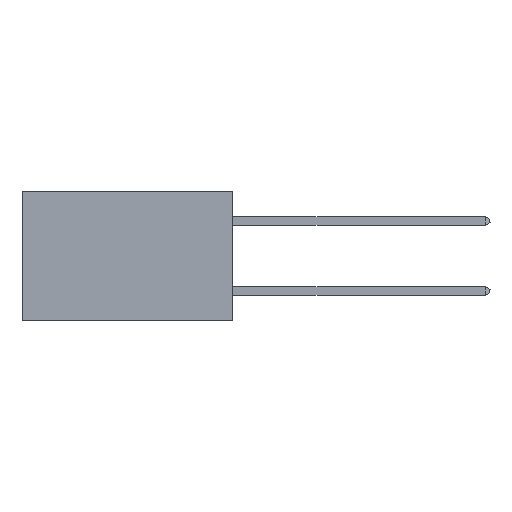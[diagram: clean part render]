
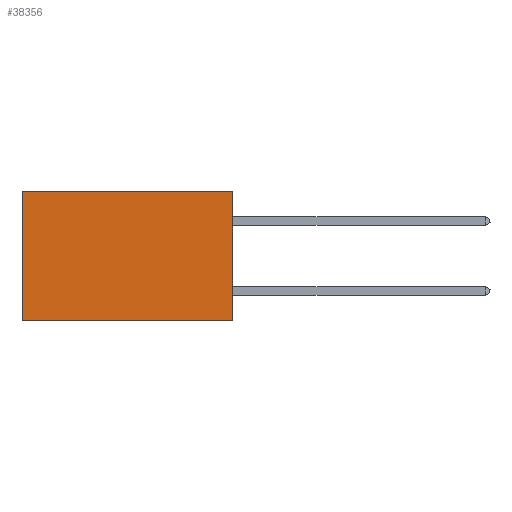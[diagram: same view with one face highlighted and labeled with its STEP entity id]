
A CAD part, left-side view. The second image highlights one B-rep face of the part: STEP entity #38356.
In plain terms, the highlighted planar face has unit normal (-1, 0, 0).
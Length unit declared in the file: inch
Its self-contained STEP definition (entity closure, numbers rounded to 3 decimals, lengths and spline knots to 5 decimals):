
#1992 = CARTESIAN_POINT ( 'NONE',  ( 0.2875, 0., -0.37 ) ) ;
#2346 = ORIENTED_EDGE ( 'NONE', *, *, #32950, .F. ) ;
#3374 = DIRECTION ( 'NONE',  ( 0., 1., 0. ) ) ;
#3600 = VECTOR ( 'NONE', #3374, 39.37008 ) ;
#3686 = VECTOR ( 'NONE', #34816, 39.37008 ) ;
#4096 = EDGE_CURVE ( 'NONE', #15948, #19096, #16349, .T. ) ;
#5787 = PLANE ( 'NONE',  #17945 ) ;
#6437 = CARTESIAN_POINT ( 'NONE',  ( 0.2875, 0., 0. ) ) ;
#8338 = VECTOR ( 'NONE', #11772, 39.37008 ) ;
#8766 = DIRECTION ( 'NONE',  ( 0., 0., -1. ) ) ;
#8863 = ORIENTED_EDGE ( 'NONE', *, *, #33765, .T. ) ;
#10231 = EDGE_CURVE ( 'NONE', #15948, #36506, #26880, .T. ) ;
#11419 = ORIENTED_EDGE ( 'NONE', *, *, #4096, .F. ) ;
#11712 = LINE ( 'NONE', #1992, #3686 ) ;
#11772 = DIRECTION ( 'NONE',  ( 0., 0., -1. ) ) ;
#11819 = CARTESIAN_POINT ( 'NONE',  ( 0.2875, 0.6, 0. ) ) ;
#15933 = VECTOR ( 'NONE', #29605, 39.37008 ) ;
#15948 = VERTEX_POINT ( 'NONE', #30671 ) ;
#16349 = LINE ( 'NONE', #17151, #8338 ) ;
#16872 = LINE ( 'NONE', #11819, #15933 ) ;
#17151 = CARTESIAN_POINT ( 'NONE',  ( 0.2875, 0., 0. ) ) ;
#17180 = ORIENTED_EDGE ( 'NONE', *, *, #10231, .T. ) ;
#17254 = CARTESIAN_POINT ( 'NONE',  ( 0.2875, 0.6, -0.37 ) ) ;
#17904 = CARTESIAN_POINT ( 'NONE',  ( 0.2875, 0., -0.37 ) ) ;
#17945 = AXIS2_PLACEMENT_3D ( 'NONE', #20693, #26630, #8766 ) ;
#19096 = VERTEX_POINT ( 'NONE', #17904 ) ;
#20693 = CARTESIAN_POINT ( 'NONE',  ( 0.2875, 0., 0. ) ) ;
#22614 = VERTEX_POINT ( 'NONE', #17254 ) ;
#24685 = CARTESIAN_POINT ( 'NONE',  ( 0.2875, 0.6, 0. ) ) ;
#25488 = FACE_OUTER_BOUND ( 'NONE', #33060, .T. ) ;
#26630 = DIRECTION ( 'NONE',  ( 1., 0., 0. ) ) ;
#26880 = LINE ( 'NONE', #6437, #3600 ) ;
#29605 = DIRECTION ( 'NONE',  ( 0., 0., -1. ) ) ;
#30671 = CARTESIAN_POINT ( 'NONE',  ( 0.2875, 0., 0. ) ) ;
#32950 = EDGE_CURVE ( 'NONE', #19096, #22614, #11712, .T. ) ;
#33060 = EDGE_LOOP ( 'NONE', ( #8863, #2346, #11419, #17180 ) ) ;
#33765 = EDGE_CURVE ( 'NONE', #36506, #22614, #16872, .T. ) ;
#34816 = DIRECTION ( 'NONE',  ( 0., 1., 0. ) ) ;
#36506 = VERTEX_POINT ( 'NONE', #24685 ) ;
#38356 = ADVANCED_FACE ( 'NONE', ( #25488 ), #5787, .F. ) ;
